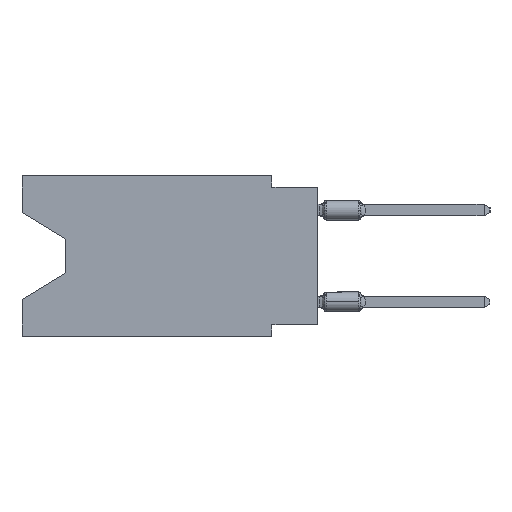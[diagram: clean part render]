
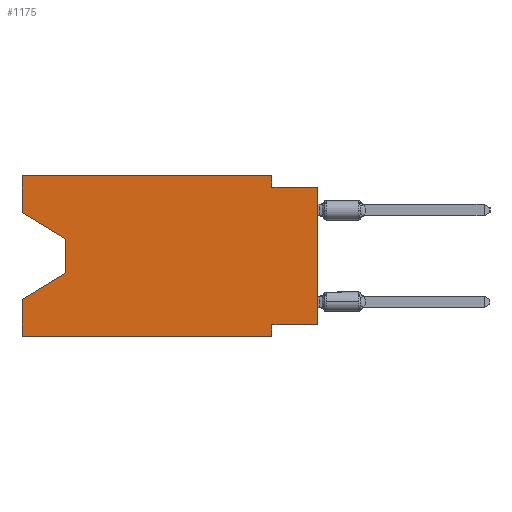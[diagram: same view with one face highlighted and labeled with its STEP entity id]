
A CAD part, left-side view. The second image highlights one B-rep face of the part: STEP entity #1175.
In plain terms, the highlighted planar face has unit normal (-1, 0, 0).
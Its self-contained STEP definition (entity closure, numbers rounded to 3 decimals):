
#11 = ORIENTED_EDGE ( 'NONE', *, *, #4413, .F. ) ;
#328 = CARTESIAN_POINT ( 'NONE',  ( 0., 0., -8.255 ) ) ;
#385 = CARTESIAN_POINT ( 'NONE',  ( 0., 0., -0.635 ) ) ;
#408 = ORIENTED_EDGE ( 'NONE', *, *, #9281, .T. ) ;
#528 = DIRECTION ( 'NONE',  ( 0., 0., 1. ) ) ;
#662 = LINE ( 'NONE', #922, #13674 ) ;
#922 = CARTESIAN_POINT ( 'NONE',  ( 0., 0., 0. ) ) ;
#1046 = FACE_OUTER_BOUND ( 'NONE', #17726, .T. ) ;
#1175 = ADVANCED_FACE ( 'NONE', ( #1046 ), #17002, .F. ) ;
#1232 = VERTEX_POINT ( 'NONE', #9032 ) ;
#1620 = VERTEX_POINT ( 'NONE', #14019 ) ;
#1735 = LINE ( 'NONE', #23547, #8599 ) ;
#2071 = LINE ( 'NONE', #328, #4515 ) ;
#2290 = DIRECTION ( 'NONE',  ( 0., 0., -1. ) ) ;
#2520 = ORIENTED_EDGE ( 'NONE', *, *, #11680, .T. ) ;
#2880 = LINE ( 'NONE', #18961, #3457 ) ;
#2907 = DIRECTION ( 'NONE',  ( 1., 0., 0. ) ) ;
#2910 = CARTESIAN_POINT ( 'NONE',  ( 0., 16.383, 0. ) ) ;
#3174 = DIRECTION ( 'NONE',  ( 0., 0., -1. ) ) ;
#3457 = VECTOR ( 'NONE', #13119, 1000. ) ;
#4413 = EDGE_CURVE ( 'NONE', #25331, #1620, #5433, .T. ) ;
#4515 = VECTOR ( 'NONE', #10319, 1000. ) ;
#4620 = LINE ( 'NONE', #25076, #18336 ) ;
#4781 = CARTESIAN_POINT ( 'NONE',  ( 0., 13.97, -3.505 ) ) ;
#5268 = CARTESIAN_POINT ( 'NONE',  ( 0., 16.383, 0. ) ) ;
#5433 = LINE ( 'NONE', #2910, #7385 ) ;
#5586 = LINE ( 'NONE', #7449, #17492 ) ;
#5640 = VECTOR ( 'NONE', #25281, 1000. ) ;
#6151 = DIRECTION ( 'NONE',  ( 0., 0.855, -0.519 ) ) ;
#6782 = VERTEX_POINT ( 'NONE', #19131 ) ;
#6823 = ORIENTED_EDGE ( 'NONE', *, *, #22605, .T. ) ;
#7038 = DIRECTION ( 'NONE',  ( 0., -1., 0. ) ) ;
#7212 = CARTESIAN_POINT ( 'NONE',  ( 0., 2.54, -8.255 ) ) ;
#7365 = EDGE_CURVE ( 'NONE', #24107, #9226, #2071, .T. ) ;
#7385 = VECTOR ( 'NONE', #7038, 1000. ) ;
#7449 = CARTESIAN_POINT ( 'NONE',  ( 0., 16.383, 0. ) ) ;
#8129 = LINE ( 'NONE', #24862, #21743 ) ;
#8153 = ORIENTED_EDGE ( 'NONE', *, *, #21718, .F. ) ;
#8201 = VECTOR ( 'NONE', #23769, 1000. ) ;
#8279 = VERTEX_POINT ( 'NONE', #385 ) ;
#8599 = VECTOR ( 'NONE', #9862, 1000. ) ;
#9032 = CARTESIAN_POINT ( 'NONE',  ( 0., 16.383, -8.89 ) ) ;
#9226 = VERTEX_POINT ( 'NONE', #7212 ) ;
#9281 = EDGE_CURVE ( 'NONE', #21116, #13321, #14926, .T. ) ;
#9399 = EDGE_CURVE ( 'NONE', #21116, #25331, #1735, .T. ) ;
#9698 = LINE ( 'NONE', #21650, #8201 ) ;
#9787 = EDGE_CURVE ( 'NONE', #9226, #6782, #9698, .T. ) ;
#9862 = DIRECTION ( 'NONE',  ( 0., 0., 1. ) ) ;
#10319 = DIRECTION ( 'NONE',  ( 0., 1., 0. ) ) ;
#10384 = CARTESIAN_POINT ( 'NONE',  ( 0., 16.383, -2.038 ) ) ;
#11070 = CARTESIAN_POINT ( 'NONE',  ( 0., 16.383, -2.038 ) ) ;
#11091 = ORIENTED_EDGE ( 'NONE', *, *, #7365, .F. ) ;
#11680 = EDGE_CURVE ( 'NONE', #13321, #21832, #16380, .T. ) ;
#12288 = VERTEX_POINT ( 'NONE', #18160 ) ;
#12703 = EDGE_CURVE ( 'NONE', #21832, #12288, #13761, .T. ) ;
#13119 = DIRECTION ( 'NONE',  ( 0., -1., 0. ) ) ;
#13321 = VERTEX_POINT ( 'NONE', #4781 ) ;
#13674 = VECTOR ( 'NONE', #528, 1000. ) ;
#13761 = LINE ( 'NONE', #21845, #24955 ) ;
#13810 = ORIENTED_EDGE ( 'NONE', *, *, #9787, .F. ) ;
#14019 = CARTESIAN_POINT ( 'NONE',  ( 0., 2.54, 0. ) ) ;
#14253 = DIRECTION ( 'NONE',  ( 0., -1., 0. ) ) ;
#14678 = ORIENTED_EDGE ( 'NONE', *, *, #16932, .F. ) ;
#14721 = CARTESIAN_POINT ( 'NONE',  ( 0., 0., -8.255 ) ) ;
#14926 = LINE ( 'NONE', #11070, #5640 ) ;
#15069 = AXIS2_PLACEMENT_3D ( 'NONE', #23358, #2907, #3174 ) ;
#16380 = LINE ( 'NONE', #22356, #22507 ) ;
#16495 = ORIENTED_EDGE ( 'NONE', *, *, #12703, .T. ) ;
#16721 = DIRECTION ( 'NONE',  ( 0., 0., -1. ) ) ;
#16932 = EDGE_CURVE ( 'NONE', #1232, #12288, #5586, .T. ) ;
#17002 = PLANE ( 'NONE',  #15069 ) ;
#17492 = VECTOR ( 'NONE', #17543, 1000. ) ;
#17543 = DIRECTION ( 'NONE',  ( 0., 0., 1. ) ) ;
#17726 = EDGE_LOOP ( 'NONE', ( #408, #2520, #16495, #14678, #19742, #13810, #11091, #6823, #24784, #8153, #11, #19286 ) ) ;
#18160 = CARTESIAN_POINT ( 'NONE',  ( 0., 16.383, -6.852 ) ) ;
#18336 = VECTOR ( 'NONE', #16721, 1000. ) ;
#18961 = CARTESIAN_POINT ( 'NONE',  ( 0., 16.383, -8.89 ) ) ;
#19131 = CARTESIAN_POINT ( 'NONE',  ( 0., 2.54, -8.89 ) ) ;
#19286 = ORIENTED_EDGE ( 'NONE', *, *, #9399, .F. ) ;
#19742 = ORIENTED_EDGE ( 'NONE', *, *, #25171, .T. ) ;
#20380 = VERTEX_POINT ( 'NONE', #24250 ) ;
#21116 = VERTEX_POINT ( 'NONE', #10384 ) ;
#21650 = CARTESIAN_POINT ( 'NONE',  ( 0., 2.54, -8.89 ) ) ;
#21718 = EDGE_CURVE ( 'NONE', #1620, #20380, #4620, .T. ) ;
#21743 = VECTOR ( 'NONE', #14253, 1000. ) ;
#21832 = VERTEX_POINT ( 'NONE', #23479 ) ;
#21845 = CARTESIAN_POINT ( 'NONE',  ( 0., 13.97, -5.385 ) ) ;
#22356 = CARTESIAN_POINT ( 'NONE',  ( 0., 13.97, -3.505 ) ) ;
#22507 = VECTOR ( 'NONE', #2290, 1000. ) ;
#22605 = EDGE_CURVE ( 'NONE', #24107, #8279, #662, .T. ) ;
#23126 = EDGE_CURVE ( 'NONE', #20380, #8279, #8129, .T. ) ;
#23358 = CARTESIAN_POINT ( 'NONE',  ( 0., 16.383, 0. ) ) ;
#23479 = CARTESIAN_POINT ( 'NONE',  ( 0., 13.97, -5.385 ) ) ;
#23547 = CARTESIAN_POINT ( 'NONE',  ( 0., 16.383, 0. ) ) ;
#23769 = DIRECTION ( 'NONE',  ( 0., 0., -1. ) ) ;
#24107 = VERTEX_POINT ( 'NONE', #14721 ) ;
#24250 = CARTESIAN_POINT ( 'NONE',  ( 0., 2.54, -0.635 ) ) ;
#24784 = ORIENTED_EDGE ( 'NONE', *, *, #23126, .F. ) ;
#24862 = CARTESIAN_POINT ( 'NONE',  ( 0., 0., -0.635 ) ) ;
#24955 = VECTOR ( 'NONE', #6151, 1000. ) ;
#25076 = CARTESIAN_POINT ( 'NONE',  ( 0., 2.54, 0. ) ) ;
#25171 = EDGE_CURVE ( 'NONE', #1232, #6782, #2880, .T. ) ;
#25281 = DIRECTION ( 'NONE',  ( 0., -0.855, -0.519 ) ) ;
#25331 = VERTEX_POINT ( 'NONE', #5268 ) ;
